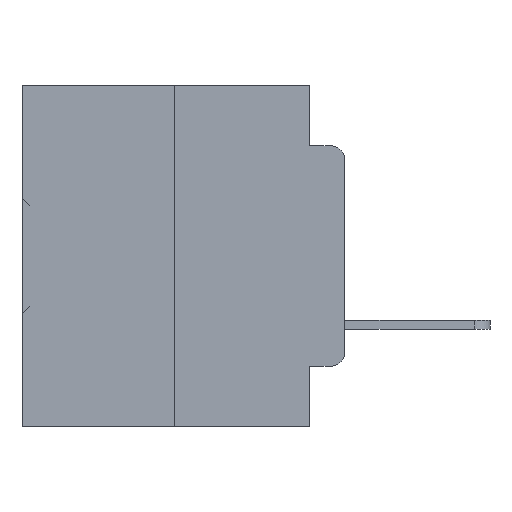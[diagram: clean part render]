
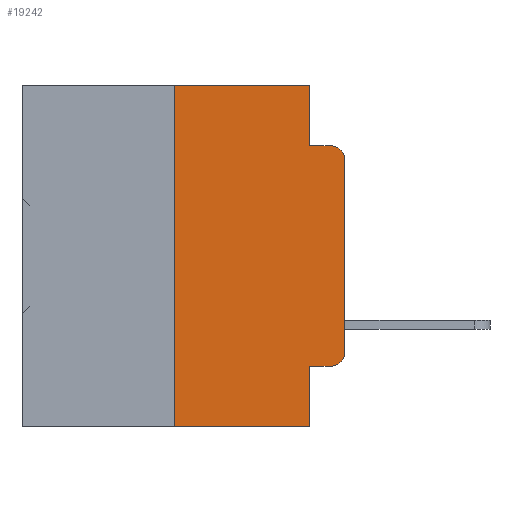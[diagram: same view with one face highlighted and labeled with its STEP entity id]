
A CAD part, left-side view. The second image highlights one B-rep face of the part: STEP entity #19242.
In plain terms, the highlighted planar face has unit normal (-1, 0, 0).
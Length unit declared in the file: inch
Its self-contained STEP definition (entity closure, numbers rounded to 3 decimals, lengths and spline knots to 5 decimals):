
#1 = VECTOR ( 'NONE', #11304, 39.37008 ) ;
#50 = ORIENTED_EDGE ( 'NONE', *, *, #13287, .T. ) ;
#1065 = CARTESIAN_POINT ( 'NONE',  ( 0., 0., 0. ) ) ;
#1334 = DIRECTION ( 'NONE',  ( 0., 0., 1. ) ) ;
#1578 = DIRECTION ( 'NONE',  ( 0., 0., -1. ) ) ;
#1900 = CARTESIAN_POINT ( 'NONE',  ( 0., 0.051, 0. ) ) ;
#2563 = CARTESIAN_POINT ( 'NONE',  ( 0., 0.25, -0.5 ) ) ;
#2795 = DIRECTION ( 'NONE',  ( 0., 0., -1. ) ) ;
#3688 = ORIENTED_EDGE ( 'NONE', *, *, #13249, .F. ) ;
#3782 = VECTOR ( 'NONE', #32734, 39.37008 ) ;
#4271 = EDGE_CURVE ( 'NONE', #35917, #19962, #12729, .T. ) ;
#4349 = CARTESIAN_POINT ( 'NONE',  ( 0., 0.051, -0.4115 ) ) ;
#4418 = VERTEX_POINT ( 'NONE', #38650 ) ;
#5031 = CARTESIAN_POINT ( 'NONE',  ( 0., 0.02, -0.0885 ) ) ;
#6329 = DIRECTION ( 'NONE',  ( 1., 0., 0. ) ) ;
#7681 = DIRECTION ( 'NONE',  ( -1., 0., 0. ) ) ;
#7685 = ORIENTED_EDGE ( 'NONE', *, *, #21908, .F. ) ;
#7727 = ORIENTED_EDGE ( 'NONE', *, *, #8638, .T. ) ;
#8442 = EDGE_CURVE ( 'NONE', #17154, #11406, #34707, .T. ) ;
#8505 = VECTOR ( 'NONE', #28133, 39.37008 ) ;
#8526 = CARTESIAN_POINT ( 'NONE',  ( 0., 0.051, -0.4115 ) ) ;
#8638 = EDGE_CURVE ( 'NONE', #15488, #4418, #25137, .T. ) ;
#10814 = CARTESIAN_POINT ( 'NONE',  ( 0., 0., -0.3915 ) ) ;
#10841 = VERTEX_POINT ( 'NONE', #22282 ) ;
#10906 = EDGE_CURVE ( 'NONE', #31769, #17154, #23398, .T. ) ;
#11304 = DIRECTION ( 'NONE',  ( 0., -1., 0. ) ) ;
#11406 = VERTEX_POINT ( 'NONE', #5031 ) ;
#11949 = DIRECTION ( 'NONE',  ( -1., 0., 0. ) ) ;
#12729 = LINE ( 'NONE', #33649, #15097 ) ;
#12773 = LINE ( 'NONE', #34223, #36527 ) ;
#13249 = EDGE_CURVE ( 'NONE', #27270, #10841, #12773, .T. ) ;
#13287 = EDGE_CURVE ( 'NONE', #4418, #31769, #21799, .T. ) ;
#13431 = EDGE_CURVE ( 'NONE', #17650, #11406, #31315, .T. ) ;
#13494 = CARTESIAN_POINT ( 'NONE',  ( 0., 0., -0.1085 ) ) ;
#13758 = CARTESIAN_POINT ( 'NONE',  ( 0., 0.02, -0.3915 ) ) ;
#14821 = VECTOR ( 'NONE', #1334, 39.37008 ) ;
#15097 = VECTOR ( 'NONE', #27922, 39.37008 ) ;
#15204 = DIRECTION ( 'NONE',  ( 0., 0., -1. ) ) ;
#15488 = VERTEX_POINT ( 'NONE', #4349 ) ;
#16291 = ORIENTED_EDGE ( 'NONE', *, *, #4271, .T. ) ;
#16618 = AXIS2_PLACEMENT_3D ( 'NONE', #27535, #6329, #15204 ) ;
#16985 = ORIENTED_EDGE ( 'NONE', *, *, #10906, .T. ) ;
#17154 = VERTEX_POINT ( 'NONE', #13494 ) ;
#17650 = VERTEX_POINT ( 'NONE', #19425 ) ;
#17914 = CARTESIAN_POINT ( 'NONE',  ( 0., 0.02, -0.1085 ) ) ;
#17999 = VECTOR ( 'NONE', #23113, 39.37008 ) ;
#18953 = DIRECTION ( 'NONE',  ( 0., -1., 0. ) ) ;
#19242 = ADVANCED_FACE ( 'NONE', ( #19446 ), #24333, .F. ) ;
#19425 = CARTESIAN_POINT ( 'NONE',  ( 0., 0.051, -0.0885 ) ) ;
#19446 = FACE_OUTER_BOUND ( 'NONE', #29640, .T. ) ;
#19962 = VERTEX_POINT ( 'NONE', #22432 ) ;
#20623 = CARTESIAN_POINT ( 'NONE',  ( 0., 0.051, -0.0885 ) ) ;
#21799 = CIRCLE ( 'NONE', #31405, 0.02 ) ;
#21908 = EDGE_CURVE ( 'NONE', #35917, #27270, #32481, .T. ) ;
#22153 = CARTESIAN_POINT ( 'NONE',  ( 0., 0.051, 0. ) ) ;
#22282 = CARTESIAN_POINT ( 'NONE',  ( 0., 0.051, 0. ) ) ;
#22432 = CARTESIAN_POINT ( 'NONE',  ( 0., 0.051, -0.5 ) ) ;
#23113 = DIRECTION ( 'NONE',  ( 0., 0., -1. ) ) ;
#23398 = LINE ( 'NONE', #1065, #14821 ) ;
#24333 = PLANE ( 'NONE',  #16618 ) ;
#24367 = VECTOR ( 'NONE', #34654, 39.37008 ) ;
#25137 = LINE ( 'NONE', #8526, #1 ) ;
#25600 = CARTESIAN_POINT ( 'NONE',  ( 0., 0.25, 0. ) ) ;
#27270 = VERTEX_POINT ( 'NONE', #35977 ) ;
#27535 = CARTESIAN_POINT ( 'NONE',  ( 0., 0.473, 0. ) ) ;
#27845 = ORIENTED_EDGE ( 'NONE', *, *, #13431, .F. ) ;
#27922 = DIRECTION ( 'NONE',  ( 0., -1., 0. ) ) ;
#28133 = DIRECTION ( 'NONE',  ( 0., 0., -1. ) ) ;
#29630 = ORIENTED_EDGE ( 'NONE', *, *, #8442, .T. ) ;
#29640 = EDGE_LOOP ( 'NONE', ( #16985, #29630, #27845, #30499, #3688, #7685, #16291, #34872, #7727, #50 ) ) ;
#30499 = ORIENTED_EDGE ( 'NONE', *, *, #38704, .F. ) ;
#30519 = AXIS2_PLACEMENT_3D ( 'NONE', #17914, #11949, #2795 ) ;
#31315 = LINE ( 'NONE', #20623, #3782 ) ;
#31405 = AXIS2_PLACEMENT_3D ( 'NONE', #13758, #7681, #1578 ) ;
#31769 = VERTEX_POINT ( 'NONE', #10814 ) ;
#32481 = LINE ( 'NONE', #25600, #24367 ) ;
#32734 = DIRECTION ( 'NONE',  ( 0., -1., 0. ) ) ;
#33177 = LINE ( 'NONE', #22153, #8505 ) ;
#33649 = CARTESIAN_POINT ( 'NONE',  ( 0., 0.473, -0.5 ) ) ;
#34172 = LINE ( 'NONE', #1900, #17999 ) ;
#34223 = CARTESIAN_POINT ( 'NONE',  ( 0., 0.473, 0. ) ) ;
#34654 = DIRECTION ( 'NONE',  ( 0., 0., 1. ) ) ;
#34707 = CIRCLE ( 'NONE', #30519, 0.02 ) ;
#34872 = ORIENTED_EDGE ( 'NONE', *, *, #39041, .F. ) ;
#35917 = VERTEX_POINT ( 'NONE', #2563 ) ;
#35977 = CARTESIAN_POINT ( 'NONE',  ( 0., 0.25, 0. ) ) ;
#36527 = VECTOR ( 'NONE', #18953, 39.37008 ) ;
#38650 = CARTESIAN_POINT ( 'NONE',  ( 0., 0.02, -0.4115 ) ) ;
#38704 = EDGE_CURVE ( 'NONE', #10841, #17650, #34172, .T. ) ;
#39041 = EDGE_CURVE ( 'NONE', #15488, #19962, #33177, .T. ) ;
